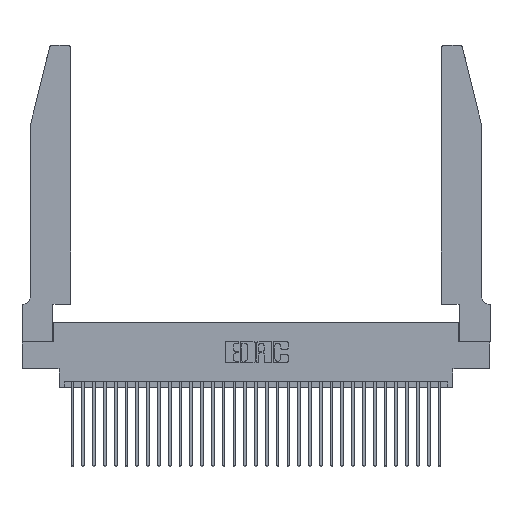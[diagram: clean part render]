
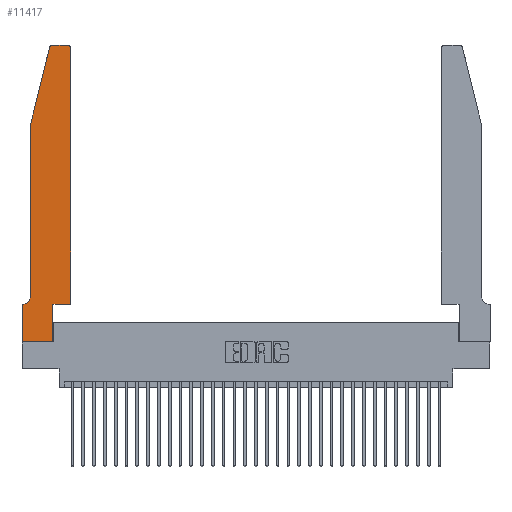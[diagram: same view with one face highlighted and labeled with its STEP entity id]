
A CAD part, top view. The second image highlights one B-rep face of the part: STEP entity #11417.
In plain terms, the highlighted planar face has unit normal (0, 0, 1).
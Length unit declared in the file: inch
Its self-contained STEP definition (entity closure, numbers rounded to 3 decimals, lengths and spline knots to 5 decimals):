
#67 = DIRECTION ( 'NONE',  ( 1., 0., 0. ) ) ;
#244 = EDGE_CURVE ( 'NONE', #5698, #6035, #15905, .T. ) ;
#445 = LINE ( 'NONE', #30193, #16107 ) ;
#486 = VECTOR ( 'NONE', #24702, 39.37008 ) ;
#1476 = EDGE_CURVE ( 'NONE', #19222, #28542, #18216, .T. ) ;
#1841 = CARTESIAN_POINT ( 'NONE',  ( 0., 0., 0.37 ) ) ;
#1875 = VERTEX_POINT ( 'NONE', #19343 ) ;
#2350 = ORIENTED_EDGE ( 'NONE', *, *, #3881, .T. ) ;
#2919 = CARTESIAN_POINT ( 'NONE',  ( 0., 0.35, 0.37 ) ) ;
#3080 = EDGE_LOOP ( 'NONE', ( #10323, #21384, #29969, #12187, #28153, #3947, #2350, #25627, #27736, #20987, #10754, #5403 ) ) ;
#3357 = CARTESIAN_POINT ( 'NONE',  ( 0.4505, 0.35, 0.37 ) ) ;
#3672 = VECTOR ( 'NONE', #16119, 39.37008 ) ;
#3841 = CARTESIAN_POINT ( 'NONE',  ( 0.2605, 2.75, 0.37 ) ) ;
#3881 = EDGE_CURVE ( 'NONE', #28542, #5698, #445, .T. ) ;
#3947 = ORIENTED_EDGE ( 'NONE', *, *, #1476, .T. ) ;
#4405 = CARTESIAN_POINT ( 'NONE',  ( 0.284, 2.75, 0.37 ) ) ;
#4664 = VERTEX_POINT ( 'NONE', #6949 ) ;
#5370 = CARTESIAN_POINT ( 'NONE',  ( 0.0755, 2., 0.37 ) ) ;
#5403 = ORIENTED_EDGE ( 'NONE', *, *, #22254, .T. ) ;
#5414 = LINE ( 'NONE', #13450, #25141 ) ;
#5551 = VERTEX_POINT ( 'NONE', #6325 ) ;
#5589 = EDGE_CURVE ( 'NONE', #4664, #9024, #19928, .T. ) ;
#5698 = VERTEX_POINT ( 'NONE', #1841 ) ;
#5806 = CARTESIAN_POINT ( 'NONE',  ( 0.0755, 2., 0.37 ) ) ;
#6035 = VERTEX_POINT ( 'NONE', #7389 ) ;
#6182 = VECTOR ( 'NONE', #12583, 39.37008 ) ;
#6325 = CARTESIAN_POINT ( 'NONE',  ( 0.0755, 2., 0.37 ) ) ;
#6661 = FACE_OUTER_BOUND ( 'NONE', #3080, .T. ) ;
#6949 = CARTESIAN_POINT ( 'NONE',  ( 0.4205, 2.75, 0.37 ) ) ;
#7389 = CARTESIAN_POINT ( 'NONE',  ( 0.2865, 0., 0.37 ) ) ;
#7579 = CARTESIAN_POINT ( 'NONE',  ( 0., 0., 0.37 ) ) ;
#9024 = VERTEX_POINT ( 'NONE', #4405 ) ;
#9623 = VERTEX_POINT ( 'NONE', #19511 ) ;
#10161 = DIRECTION ( 'NONE',  ( 0., 0., 1. ) ) ;
#10212 = EDGE_CURVE ( 'NONE', #5551, #11632, #28128, .T. ) ;
#10285 = VERTEX_POINT ( 'NONE', #3357 ) ;
#10323 = ORIENTED_EDGE ( 'NONE', *, *, #5589, .T. ) ;
#10754 = ORIENTED_EDGE ( 'NONE', *, *, #23386, .T. ) ;
#11006 = CARTESIAN_POINT ( 'NONE',  ( 0.0755, 0.42, 0.37 ) ) ;
#11417 = ADVANCED_FACE ( 'NONE', ( #6661 ), #18133, .T. ) ;
#11632 = VERTEX_POINT ( 'NONE', #11006 ) ;
#12042 = DIRECTION ( 'NONE',  ( 0., 0., -1. ) ) ;
#12187 = ORIENTED_EDGE ( 'NONE', *, *, #10212, .T. ) ;
#12395 = LINE ( 'NONE', #30351, #29377 ) ;
#12583 = DIRECTION ( 'NONE',  ( -1., 0., 0. ) ) ;
#12674 = VECTOR ( 'NONE', #21853, 39.37008 ) ;
#12912 = CARTESIAN_POINT ( 'NONE',  ( 0.0055, 0.35, 0.37 ) ) ;
#13035 = DIRECTION ( 'NONE',  ( 1., 0., 0. ) ) ;
#13388 = EDGE_CURVE ( 'NONE', #11632, #19222, #23156, .T. ) ;
#13450 = CARTESIAN_POINT ( 'NONE',  ( 0.4505, 0.35, 0.37 ) ) ;
#13562 = DIRECTION ( 'NONE',  ( 0., 1., 0. ) ) ;
#14616 = DIRECTION ( 'NONE',  ( -1., 0., 0. ) ) ;
#14847 = DIRECTION ( 'NONE',  ( 1., 0., 0. ) ) ;
#15117 = DIRECTION ( 'NONE',  ( 1., 0., 0. ) ) ;
#15444 = EDGE_CURVE ( 'NONE', #1875, #5551, #20166, .T. ) ;
#15624 = DIRECTION ( 'NONE',  ( 0., -1., 0. ) ) ;
#15627 = EDGE_CURVE ( 'NONE', #6035, #16627, #15721, .T. ) ;
#15721 = LINE ( 'NONE', #21753, #486 ) ;
#15905 = LINE ( 'NONE', #7579, #33276 ) ;
#16107 = VECTOR ( 'NONE', #19884, 39.37008 ) ;
#16119 = DIRECTION ( 'NONE',  ( -0.239, -0.971, 0. ) ) ;
#16572 = CARTESIAN_POINT ( 'NONE',  ( 0.4205, 2.72, 0.37 ) ) ;
#16627 = VERTEX_POINT ( 'NONE', #25761 ) ;
#17805 = CARTESIAN_POINT ( 'NONE',  ( 0., 0.35, 0.37 ) ) ;
#18133 = PLANE ( 'NONE',  #18244 ) ;
#18216 = LINE ( 'NONE', #28085, #6182 ) ;
#18244 = AXIS2_PLACEMENT_3D ( 'NONE', #17805, #20764, #15117 ) ;
#19222 = VERTEX_POINT ( 'NONE', #12912 ) ;
#19343 = CARTESIAN_POINT ( 'NONE',  ( 0.25487, 2.72718, 0.37 ) ) ;
#19511 = CARTESIAN_POINT ( 'NONE',  ( 0.4505, 2.72, 0.37 ) ) ;
#19527 = DIRECTION ( 'NONE',  ( 1., 0., 0. ) ) ;
#19884 = DIRECTION ( 'NONE',  ( 0., -1., 0. ) ) ;
#19928 = LINE ( 'NONE', #3841, #12674 ) ;
#20166 = LINE ( 'NONE', #5806, #3672 ) ;
#20764 = DIRECTION ( 'NONE',  ( 0., 0., 1. ) ) ;
#20987 = ORIENTED_EDGE ( 'NONE', *, *, #32819, .T. ) ;
#21384 = ORIENTED_EDGE ( 'NONE', *, *, #30999, .T. ) ;
#21753 = CARTESIAN_POINT ( 'NONE',  ( 0.2865, 0.35, 0.37 ) ) ;
#21853 = DIRECTION ( 'NONE',  ( -1., 0., 0. ) ) ;
#22254 = EDGE_CURVE ( 'NONE', #9623, #4664, #26027, .T. ) ;
#23099 = CARTESIAN_POINT ( 'NONE',  ( 0.284, 2.72, 0.37 ) ) ;
#23156 = CIRCLE ( 'NONE', #28479, 0.07 ) ;
#23386 = EDGE_CURVE ( 'NONE', #10285, #9623, #5414, .T. ) ;
#23770 = AXIS2_PLACEMENT_3D ( 'NONE', #23099, #10161, #67 ) ;
#24702 = DIRECTION ( 'NONE',  ( 0., 1., 0. ) ) ;
#25141 = VECTOR ( 'NONE', #13562, 39.37008 ) ;
#25627 = ORIENTED_EDGE ( 'NONE', *, *, #244, .T. ) ;
#25747 = CIRCLE ( 'NONE', #23770, 0.03 ) ;
#25761 = CARTESIAN_POINT ( 'NONE',  ( 0.2865, 0.35, 0.37 ) ) ;
#26027 = CIRCLE ( 'NONE', #31152, 0.03 ) ;
#27736 = ORIENTED_EDGE ( 'NONE', *, *, #15627, .T. ) ;
#28085 = CARTESIAN_POINT ( 'NONE',  ( 0.0755, 0.35, 0.37 ) ) ;
#28128 = LINE ( 'NONE', #5370, #28930 ) ;
#28153 = ORIENTED_EDGE ( 'NONE', *, *, #13388, .T. ) ;
#28479 = AXIS2_PLACEMENT_3D ( 'NONE', #30008, #12042, #14616 ) ;
#28542 = VERTEX_POINT ( 'NONE', #2919 ) ;
#28930 = VECTOR ( 'NONE', #15624, 39.37008 ) ;
#29377 = VECTOR ( 'NONE', #14847, 39.37008 ) ;
#29969 = ORIENTED_EDGE ( 'NONE', *, *, #15444, .T. ) ;
#30008 = CARTESIAN_POINT ( 'NONE',  ( 0.0055, 0.42, 0.37 ) ) ;
#30193 = CARTESIAN_POINT ( 'NONE',  ( 0., 0., 0.37 ) ) ;
#30351 = CARTESIAN_POINT ( 'NONE',  ( 0.4505, 0.35, 0.37 ) ) ;
#30999 = EDGE_CURVE ( 'NONE', #9024, #1875, #25747, .T. ) ;
#31152 = AXIS2_PLACEMENT_3D ( 'NONE', #16572, #32515, #19527 ) ;
#32515 = DIRECTION ( 'NONE',  ( 0., 0., 1. ) ) ;
#32819 = EDGE_CURVE ( 'NONE', #16627, #10285, #12395, .T. ) ;
#33276 = VECTOR ( 'NONE', #13035, 39.37008 ) ;
